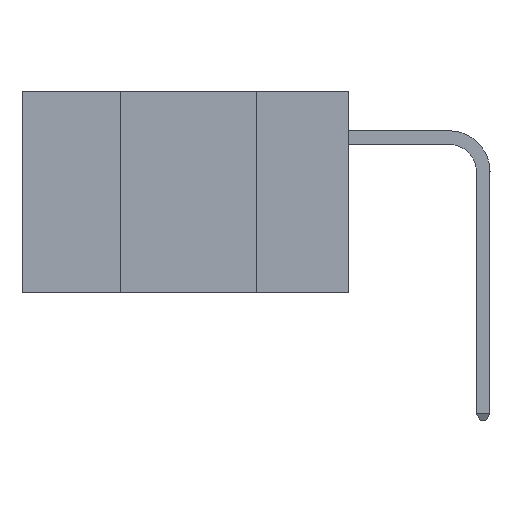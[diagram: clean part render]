
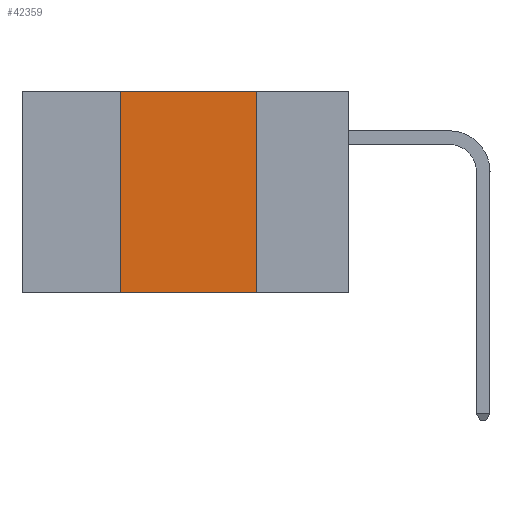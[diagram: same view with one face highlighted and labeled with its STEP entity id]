
A CAD part, left-side view. The second image highlights one B-rep face of the part: STEP entity #42359.
In plain terms, the highlighted planar face has unit normal (-1, 0, 0).
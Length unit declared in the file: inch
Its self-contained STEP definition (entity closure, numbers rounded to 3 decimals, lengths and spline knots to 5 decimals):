
#982 = VERTEX_POINT ( 'NONE', #34086 ) ;
#2510 = ORIENTED_EDGE ( 'NONE', *, *, #37561, .T. ) ;
#2834 = ORIENTED_EDGE ( 'NONE', *, *, #31029, .F. ) ;
#9722 = CARTESIAN_POINT ( 'NONE',  ( 0., 0.42, 0. ) ) ;
#10559 = VERTEX_POINT ( 'NONE', #22286 ) ;
#11998 = CARTESIAN_POINT ( 'NONE',  ( 0., 0.17, 0. ) ) ;
#13720 = CARTESIAN_POINT ( 'NONE',  ( 0., 0.6, 0. ) ) ;
#13847 = LINE ( 'NONE', #13720, #40084 ) ;
#15338 = CARTESIAN_POINT ( 'NONE',  ( 0., 0.17, -0.37 ) ) ;
#19441 = EDGE_LOOP ( 'NONE', ( #45786, #2834, #20864, #2510 ) ) ;
#19444 = DIRECTION ( 'NONE',  ( 0., 0., -1. ) ) ;
#20261 = EDGE_CURVE ( 'NONE', #982, #10559, #44587, .T. ) ;
#20864 = ORIENTED_EDGE ( 'NONE', *, *, #20261, .F. ) ;
#21417 = CARTESIAN_POINT ( 'NONE',  ( 0., 0.17, 0. ) ) ;
#22286 = CARTESIAN_POINT ( 'NONE',  ( 0., 0.42, 0. ) ) ;
#23507 = VERTEX_POINT ( 'NONE', #15338 ) ;
#26507 = VECTOR ( 'NONE', #28277, 39.37008 ) ;
#28277 = DIRECTION ( 'NONE',  ( 0., -1., 0. ) ) ;
#28860 = DIRECTION ( 'NONE',  ( 0., -1., 0. ) ) ;
#31029 = EDGE_CURVE ( 'NONE', #10559, #37605, #13847, .T. ) ;
#31259 = DIRECTION ( 'NONE',  ( 0., 0., 1. ) ) ;
#31590 = PLANE ( 'NONE',  #32221 ) ;
#31810 = CARTESIAN_POINT ( 'NONE',  ( 0., 0.6, -0.37 ) ) ;
#32221 = AXIS2_PLACEMENT_3D ( 'NONE', #38905, #39064, #38754 ) ;
#34086 = CARTESIAN_POINT ( 'NONE',  ( 0., 0.42, -0.37 ) ) ;
#35177 = EDGE_CURVE ( 'NONE', #37605, #23507, #40461, .T. ) ;
#37561 = EDGE_CURVE ( 'NONE', #982, #23507, #44267, .T. ) ;
#37605 = VERTEX_POINT ( 'NONE', #21417 ) ;
#38754 = DIRECTION ( 'NONE',  ( 0., 0., -1. ) ) ;
#38861 = VECTOR ( 'NONE', #31259, 39.37008 ) ;
#38905 = CARTESIAN_POINT ( 'NONE',  ( 0., 0.6, 0. ) ) ;
#39064 = DIRECTION ( 'NONE',  ( 1., 0., 0. ) ) ;
#40084 = VECTOR ( 'NONE', #28860, 39.37008 ) ;
#40461 = LINE ( 'NONE', #11998, #42777 ) ;
#42359 = ADVANCED_FACE ( 'NONE', ( #46340 ), #31590, .F. ) ;
#42777 = VECTOR ( 'NONE', #19444, 39.37008 ) ;
#44267 = LINE ( 'NONE', #31810, #26507 ) ;
#44587 = LINE ( 'NONE', #9722, #38861 ) ;
#45786 = ORIENTED_EDGE ( 'NONE', *, *, #35177, .F. ) ;
#46340 = FACE_OUTER_BOUND ( 'NONE', #19441, .T. ) ;
